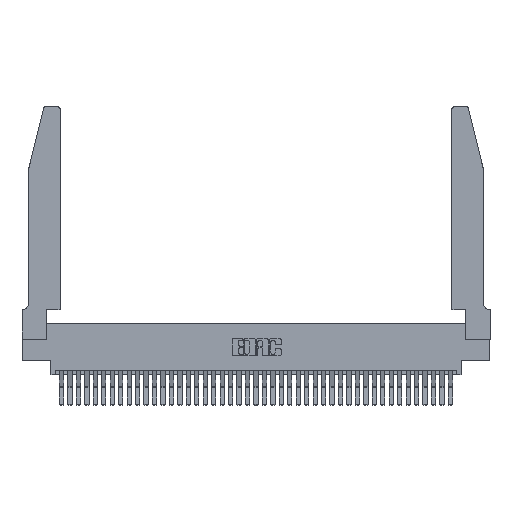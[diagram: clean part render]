
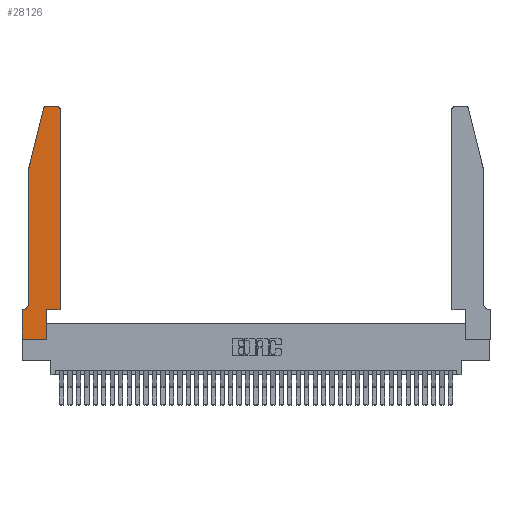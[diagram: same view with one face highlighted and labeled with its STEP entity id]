
A CAD part, top view. The second image highlights one B-rep face of the part: STEP entity #28126.
In plain terms, the highlighted planar face has unit normal (0, 0, 1).
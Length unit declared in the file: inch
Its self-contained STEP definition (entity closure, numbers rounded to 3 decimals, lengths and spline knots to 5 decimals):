
#232 = CARTESIAN_POINT ( 'NONE',  ( 0.2865, 0., 0.37 ) ) ;
#1196 = DIRECTION ( 'NONE',  ( 1., 0., 0. ) ) ;
#1574 = LINE ( 'NONE', #40105, #34451 ) ;
#1601 = FACE_OUTER_BOUND ( 'NONE', #11322, .T. ) ;
#1782 = CARTESIAN_POINT ( 'NONE',  ( 0.2865, 0.35, 0.37 ) ) ;
#2100 = EDGE_CURVE ( 'NONE', #19006, #22687, #5571, .T. ) ;
#2349 = VERTEX_POINT ( 'NONE', #19853 ) ;
#2717 = AXIS2_PLACEMENT_3D ( 'NONE', #39312, #20342, #1196 ) ;
#3130 = ORIENTED_EDGE ( 'NONE', *, *, #17968, .T. ) ;
#3443 = VERTEX_POINT ( 'NONE', #6582 ) ;
#3730 = CARTESIAN_POINT ( 'NONE',  ( 0.4205, 2.75, 0.37 ) ) ;
#3822 = DIRECTION ( 'NONE',  ( 0., 1., 0. ) ) ;
#4948 = LINE ( 'NONE', #30887, #29317 ) ;
#5441 = VECTOR ( 'NONE', #3822, 39.37008 ) ;
#5571 = LINE ( 'NONE', #31358, #28938 ) ;
#6269 = ORIENTED_EDGE ( 'NONE', *, *, #2100, .T. ) ;
#6491 = ORIENTED_EDGE ( 'NONE', *, *, #30920, .T. ) ;
#6582 = CARTESIAN_POINT ( 'NONE',  ( 0.25487, 2.72718, 0.37 ) ) ;
#6885 = ORIENTED_EDGE ( 'NONE', *, *, #36521, .T. ) ;
#7414 = VECTOR ( 'NONE', #38863, 39.37008 ) ;
#10310 = CARTESIAN_POINT ( 'NONE',  ( 0.4505, 0.35, 0.37 ) ) ;
#10420 = CIRCLE ( 'NONE', #19466, 0.03 ) ;
#11322 = EDGE_LOOP ( 'NONE', ( #6269, #32303, #22133, #26007, #6491, #18338, #6885, #24246, #38899, #3130, #35411, #38955 ) ) ;
#11551 = EDGE_CURVE ( 'NONE', #29646, #40814, #36028, .T. ) ;
#13004 = CARTESIAN_POINT ( 'NONE',  ( 0.0755, 0.42, 0.37 ) ) ;
#13419 = EDGE_CURVE ( 'NONE', #3443, #14431, #1574, .T. ) ;
#13804 = VERTEX_POINT ( 'NONE', #36343 ) ;
#14431 = VERTEX_POINT ( 'NONE', #27011 ) ;
#15277 = DIRECTION ( 'NONE',  ( 0., -1., 0. ) ) ;
#15571 = EDGE_CURVE ( 'NONE', #14431, #38729, #32777, .T. ) ;
#15949 = EDGE_CURVE ( 'NONE', #13804, #19006, #10420, .T. ) ;
#16274 = CARTESIAN_POINT ( 'NONE',  ( 0.0055, 0.42, 0.37 ) ) ;
#17333 = CARTESIAN_POINT ( 'NONE',  ( 0., 0.35, 0.37 ) ) ;
#17963 = DIRECTION ( 'NONE',  ( -0.239, -0.971, 0. ) ) ;
#17968 = EDGE_CURVE ( 'NONE', #40814, #19146, #29414, .T. ) ;
#18338 = ORIENTED_EDGE ( 'NONE', *, *, #33585, .T. ) ;
#18778 = CARTESIAN_POINT ( 'NONE',  ( 0.4205, 2.72, 0.37 ) ) ;
#19006 = VERTEX_POINT ( 'NONE', #3730 ) ;
#19146 = VERTEX_POINT ( 'NONE', #26694 ) ;
#19178 = VECTOR ( 'NONE', #30286, 39.37008 ) ;
#19428 = DIRECTION ( 'NONE',  ( -1., 0., 0. ) ) ;
#19466 = AXIS2_PLACEMENT_3D ( 'NONE', #18778, #40911, #21974 ) ;
#19732 = CARTESIAN_POINT ( 'NONE',  ( 0.4505, 0.35, 0.37 ) ) ;
#19764 = CARTESIAN_POINT ( 'NONE',  ( 0.0755, 2., 0.37 ) ) ;
#19853 = CARTESIAN_POINT ( 'NONE',  ( 0.0055, 0.35, 0.37 ) ) ;
#20342 = DIRECTION ( 'NONE',  ( 0., 0., 1. ) ) ;
#20503 = PLANE ( 'NONE',  #28507 ) ;
#20588 = DIRECTION ( 'NONE',  ( -1., 0., 0. ) ) ;
#21974 = DIRECTION ( 'NONE',  ( 1., 0., 0. ) ) ;
#22133 = ORIENTED_EDGE ( 'NONE', *, *, #13419, .T. ) ;
#22227 = AXIS2_PLACEMENT_3D ( 'NONE', #16274, #38396, #19428 ) ;
#22687 = VERTEX_POINT ( 'NONE', #26711 ) ;
#23695 = DIRECTION ( 'NONE',  ( 1., 0., 0. ) ) ;
#24246 = ORIENTED_EDGE ( 'NONE', *, *, #32265, .T. ) ;
#24606 = EDGE_CURVE ( 'NONE', #19146, #13804, #39212, .T. ) ;
#25155 = DIRECTION ( 'NONE',  ( -1., 0., 0. ) ) ;
#25532 = CARTESIAN_POINT ( 'NONE',  ( 0., 0.35, 0.37 ) ) ;
#26007 = ORIENTED_EDGE ( 'NONE', *, *, #15571, .T. ) ;
#26120 = DIRECTION ( 'NONE',  ( 1., 0., 0. ) ) ;
#26244 = DIRECTION ( 'NONE',  ( 1., 0., 0. ) ) ;
#26694 = CARTESIAN_POINT ( 'NONE',  ( 0.4505, 0.35, 0.37 ) ) ;
#26711 = CARTESIAN_POINT ( 'NONE',  ( 0.284, 2.75, 0.37 ) ) ;
#27011 = CARTESIAN_POINT ( 'NONE',  ( 0.0755, 2., 0.37 ) ) ;
#28126 = ADVANCED_FACE ( 'NONE', ( #1601 ), #20503, .T. ) ;
#28507 = AXIS2_PLACEMENT_3D ( 'NONE', #17333, #33109, #23695 ) ;
#28938 = VECTOR ( 'NONE', #25155, 39.37008 ) ;
#29317 = VECTOR ( 'NONE', #15277, 39.37008 ) ;
#29381 = LINE ( 'NONE', #39101, #37839 ) ;
#29414 = LINE ( 'NONE', #10310, #36882 ) ;
#29646 = VERTEX_POINT ( 'NONE', #232 ) ;
#30286 = DIRECTION ( 'NONE',  ( 0., 1., 0. ) ) ;
#30872 = VERTEX_POINT ( 'NONE', #25532 ) ;
#30887 = CARTESIAN_POINT ( 'NONE',  ( 0., 0., 0.37 ) ) ;
#30920 = EDGE_CURVE ( 'NONE', #38729, #2349, #35960, .T. ) ;
#31358 = CARTESIAN_POINT ( 'NONE',  ( 0.2605, 2.75, 0.37 ) ) ;
#31675 = EDGE_CURVE ( 'NONE', #22687, #3443, #33429, .T. ) ;
#31699 = CARTESIAN_POINT ( 'NONE',  ( 0., 0., 0.37 ) ) ;
#32253 = VECTOR ( 'NONE', #20588, 39.37008 ) ;
#32265 = EDGE_CURVE ( 'NONE', #35247, #29646, #29381, .T. ) ;
#32303 = ORIENTED_EDGE ( 'NONE', *, *, #31675, .T. ) ;
#32777 = LINE ( 'NONE', #19764, #7414 ) ;
#33109 = DIRECTION ( 'NONE',  ( 0., 0., 1. ) ) ;
#33194 = CARTESIAN_POINT ( 'NONE',  ( 0.0755, 0.35, 0.37 ) ) ;
#33267 = LINE ( 'NONE', #33194, #32253 ) ;
#33429 = CIRCLE ( 'NONE', #2717, 0.03 ) ;
#33466 = CARTESIAN_POINT ( 'NONE',  ( 0.2865, 0.35, 0.37 ) ) ;
#33585 = EDGE_CURVE ( 'NONE', #2349, #30872, #33267, .T. ) ;
#34451 = VECTOR ( 'NONE', #17963, 39.37008 ) ;
#35247 = VERTEX_POINT ( 'NONE', #31699 ) ;
#35411 = ORIENTED_EDGE ( 'NONE', *, *, #24606, .T. ) ;
#35960 = CIRCLE ( 'NONE', #22227, 0.07 ) ;
#36028 = LINE ( 'NONE', #1782, #19178 ) ;
#36343 = CARTESIAN_POINT ( 'NONE',  ( 0.4505, 2.72, 0.37 ) ) ;
#36521 = EDGE_CURVE ( 'NONE', #30872, #35247, #4948, .T. ) ;
#36882 = VECTOR ( 'NONE', #26120, 39.37008 ) ;
#37839 = VECTOR ( 'NONE', #26244, 39.37008 ) ;
#38396 = DIRECTION ( 'NONE',  ( 0., 0., -1. ) ) ;
#38729 = VERTEX_POINT ( 'NONE', #13004 ) ;
#38863 = DIRECTION ( 'NONE',  ( 0., -1., 0. ) ) ;
#38899 = ORIENTED_EDGE ( 'NONE', *, *, #11551, .T. ) ;
#38955 = ORIENTED_EDGE ( 'NONE', *, *, #15949, .T. ) ;
#39101 = CARTESIAN_POINT ( 'NONE',  ( 0., 0., 0.37 ) ) ;
#39212 = LINE ( 'NONE', #19732, #5441 ) ;
#39312 = CARTESIAN_POINT ( 'NONE',  ( 0.284, 2.72, 0.37 ) ) ;
#40105 = CARTESIAN_POINT ( 'NONE',  ( 0.0755, 2., 0.37 ) ) ;
#40814 = VERTEX_POINT ( 'NONE', #33466 ) ;
#40911 = DIRECTION ( 'NONE',  ( 0., 0., 1. ) ) ;
